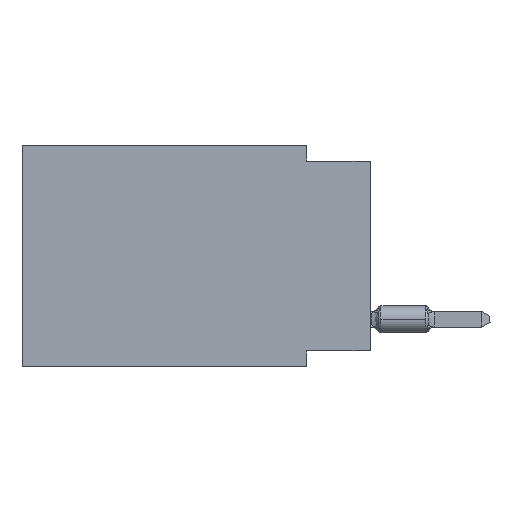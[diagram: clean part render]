
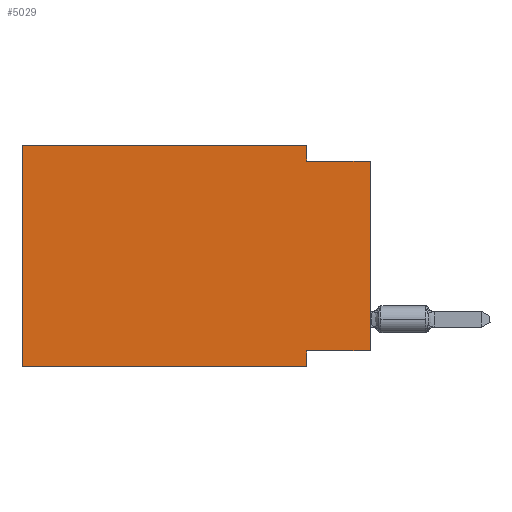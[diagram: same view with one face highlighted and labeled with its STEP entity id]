
A CAD part, left-side view. The second image highlights one B-rep face of the part: STEP entity #5029.
In plain terms, the highlighted planar face has unit normal (-1, 0, 0).
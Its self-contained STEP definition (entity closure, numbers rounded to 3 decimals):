
#790 = DIRECTION ( 'NONE',  ( 0., 1., 0. ) ) ;
#2816 = DIRECTION ( 'NONE',  ( 0., -1., 0. ) ) ;
#3507 = DIRECTION ( 'NONE',  ( 1., 0., 0. ) ) ;
#3970 = EDGE_CURVE ( 'NONE', #30114, #38003, #13867, .T. ) ;
#4060 = CARTESIAN_POINT ( 'NONE',  ( 0., 0., -0.635 ) ) ;
#5029 = ADVANCED_FACE ( 'NONE', ( #18161 ), #29953, .F. ) ;
#5048 = LINE ( 'NONE', #25869, #13719 ) ;
#5305 = EDGE_CURVE ( 'NONE', #34988, #14317, #37861, .T. ) ;
#5418 = CARTESIAN_POINT ( 'NONE',  ( 0., 13.97, -8.89 ) ) ;
#5924 = CARTESIAN_POINT ( 'NONE',  ( 0., 2.54, -8.255 ) ) ;
#6010 = VERTEX_POINT ( 'NONE', #11299 ) ;
#6484 = LINE ( 'NONE', #15716, #33400 ) ;
#6717 = CARTESIAN_POINT ( 'NONE',  ( 0., 0., 0. ) ) ;
#7371 = VERTEX_POINT ( 'NONE', #14734 ) ;
#8783 = CARTESIAN_POINT ( 'NONE',  ( 0., 0., -0.635 ) ) ;
#9258 = ORIENTED_EDGE ( 'NONE', *, *, #14380, .F. ) ;
#9567 = EDGE_CURVE ( 'NONE', #7371, #30114, #13368, .T. ) ;
#10126 = DIRECTION ( 'NONE',  ( 0., -1., 0. ) ) ;
#10593 = ORIENTED_EDGE ( 'NONE', *, *, #29032, .F. ) ;
#10745 = ORIENTED_EDGE ( 'NONE', *, *, #9567, .F. ) ;
#11299 = CARTESIAN_POINT ( 'NONE',  ( 0., 2.54, -8.89 ) ) ;
#12761 = ORIENTED_EDGE ( 'NONE', *, *, #3970, .F. ) ;
#13128 = CARTESIAN_POINT ( 'NONE',  ( 0., 13.97, 0. ) ) ;
#13368 = LINE ( 'NONE', #25130, #14213 ) ;
#13719 = VECTOR ( 'NONE', #14097, 1000. ) ;
#13867 = LINE ( 'NONE', #33940, #30813 ) ;
#13976 = CARTESIAN_POINT ( 'NONE',  ( 0., 2.54, -0.635 ) ) ;
#14097 = DIRECTION ( 'NONE',  ( 0., 0., 1. ) ) ;
#14213 = VECTOR ( 'NONE', #36932, 1000. ) ;
#14317 = VERTEX_POINT ( 'NONE', #4060 ) ;
#14380 = EDGE_CURVE ( 'NONE', #34988, #18450, #15423, .T. ) ;
#14734 = CARTESIAN_POINT ( 'NONE',  ( 0., 13.97, 0. ) ) ;
#15423 = LINE ( 'NONE', #17946, #16534 ) ;
#15486 = ORIENTED_EDGE ( 'NONE', *, *, #32649, .F. ) ;
#15610 = CARTESIAN_POINT ( 'NONE',  ( 0., 0., -8.255 ) ) ;
#15685 = CARTESIAN_POINT ( 'NONE',  ( 0., 2.54, 0. ) ) ;
#15716 = CARTESIAN_POINT ( 'NONE',  ( 0., 13.97, -8.89 ) ) ;
#16188 = DIRECTION ( 'NONE',  ( 0., 0., -1. ) ) ;
#16534 = VECTOR ( 'NONE', #790, 1000. ) ;
#17946 = CARTESIAN_POINT ( 'NONE',  ( 0., 0., -8.255 ) ) ;
#18161 = FACE_OUTER_BOUND ( 'NONE', #34312, .T. ) ;
#18450 = VERTEX_POINT ( 'NONE', #5924 ) ;
#19918 = EDGE_CURVE ( 'NONE', #28266, #7371, #5048, .T. ) ;
#23416 = ORIENTED_EDGE ( 'NONE', *, *, #25213, .T. ) ;
#23626 = LINE ( 'NONE', #8783, #35196 ) ;
#24673 = CARTESIAN_POINT ( 'NONE',  ( 0., 2.54, -8.89 ) ) ;
#24689 = DIRECTION ( 'NONE',  ( 0., 0., -1. ) ) ;
#25109 = ORIENTED_EDGE ( 'NONE', *, *, #5305, .T. ) ;
#25130 = CARTESIAN_POINT ( 'NONE',  ( 0., 13.97, 0. ) ) ;
#25213 = EDGE_CURVE ( 'NONE', #28266, #6010, #6484, .T. ) ;
#25869 = CARTESIAN_POINT ( 'NONE',  ( 0., 13.97, 0. ) ) ;
#26052 = DIRECTION ( 'NONE',  ( 0., 0., 1. ) ) ;
#27586 = LINE ( 'NONE', #24673, #28113 ) ;
#27790 = VECTOR ( 'NONE', #26052, 1000. ) ;
#28113 = VECTOR ( 'NONE', #16188, 1000. ) ;
#28266 = VERTEX_POINT ( 'NONE', #5418 ) ;
#28329 = DIRECTION ( 'NONE',  ( 0., 0., -1. ) ) ;
#29032 = EDGE_CURVE ( 'NONE', #38003, #14317, #23626, .T. ) ;
#29953 = PLANE ( 'NONE',  #30293 ) ;
#30114 = VERTEX_POINT ( 'NONE', #15685 ) ;
#30293 = AXIS2_PLACEMENT_3D ( 'NONE', #13128, #3507, #24689 ) ;
#30813 = VECTOR ( 'NONE', #28329, 1000. ) ;
#31619 = ORIENTED_EDGE ( 'NONE', *, *, #19918, .F. ) ;
#32649 = EDGE_CURVE ( 'NONE', #18450, #6010, #27586, .T. ) ;
#33400 = VECTOR ( 'NONE', #10126, 1000. ) ;
#33940 = CARTESIAN_POINT ( 'NONE',  ( 0., 2.54, 0. ) ) ;
#34312 = EDGE_LOOP ( 'NONE', ( #25109, #10593, #12761, #10745, #31619, #23416, #15486, #9258 ) ) ;
#34988 = VERTEX_POINT ( 'NONE', #15610 ) ;
#35196 = VECTOR ( 'NONE', #2816, 1000. ) ;
#36932 = DIRECTION ( 'NONE',  ( 0., -1., 0. ) ) ;
#37861 = LINE ( 'NONE', #6717, #27790 ) ;
#38003 = VERTEX_POINT ( 'NONE', #13976 ) ;
